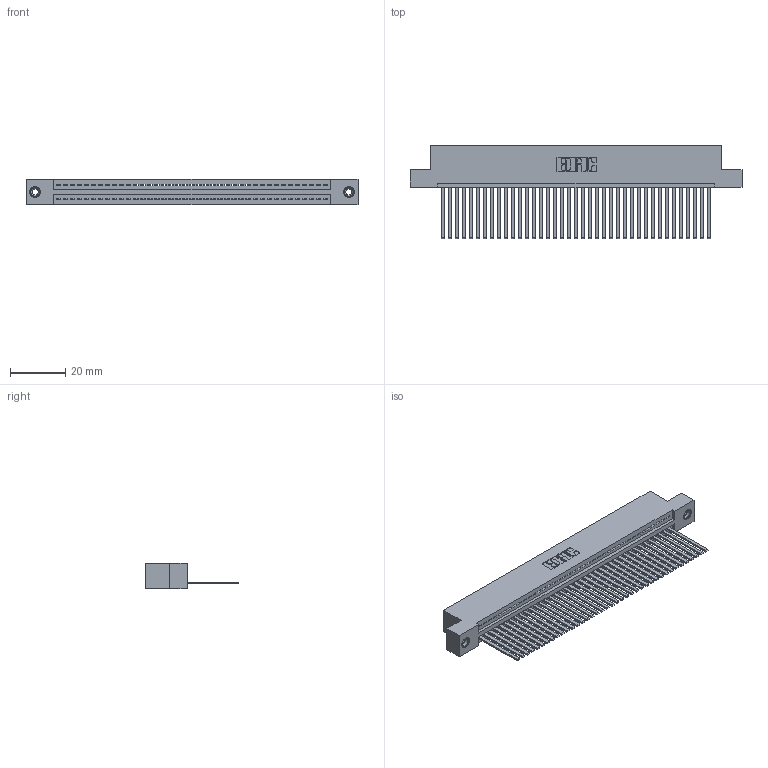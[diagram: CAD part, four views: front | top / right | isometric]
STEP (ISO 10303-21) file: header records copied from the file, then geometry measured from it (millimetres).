
FILE_DESCRIPTION (( 'STEP AP203' ), '1' );
FILE_NAME ('345-039-544-108.STEP', '2018-09-04T23:37:46', ( '' ), ( '' ), 'SwSTEP 2.0', 'SolidWorks 2016', '' );
FILE_SCHEMA (( 'CONFIG_CONTROL_DESIGN' ));
Length unit declared in the file: inch
Products named in the file (4): 345-039-544-108; 345 Part_Flush Mounting Lugs - 0.156 Dia-TI; 345-292-001_345-293-144; 345-250-001_345-250-003-102
Assembly tree (42 placements, depth 2):
  345-039-544-108
    345 Part_Flush Mounting Lugs - 0.156 Dia-TI
    345-292-001_345-293-144  x39
    345-250-001_345-250-003-102  x2
Bounding box: 120.27 x 33.96 x 9.4 mm (x, y, z)
Volume: 11843.8 mm3; surface area: 17073.8 mm2
Topology: 42 solids, 42 shells, 2214 faces, 6639 edges, 4366 vertices
Faces by surface type: plane 1516, cylinder 682, cone 12, torus 4
Entity records: 30758 total; most frequent: CARTESIAN_POINT 5308, ORIENTED_EDGE 5274, DIRECTION 4665, EDGE_CURVE 2637, LINE 2333, VECTOR 2333, VERTEX_POINT 1752, AXIS2_PLACEMENT_3D 1166
